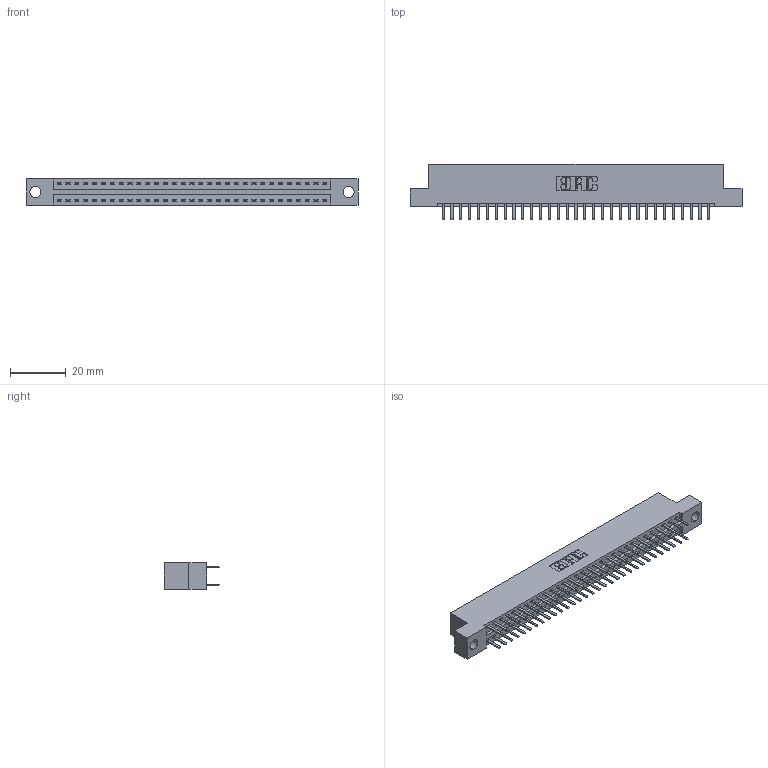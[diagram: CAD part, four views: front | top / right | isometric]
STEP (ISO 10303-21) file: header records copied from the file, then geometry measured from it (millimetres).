
FILE_DESCRIPTION (( 'STEP AP203' ), '1' );
FILE_NAME ('346-062-520-204.STEP', '2022-05-24T13:14:54', ( '' ), ( '' ), 'SwSTEP 2.0', 'SolidWorks 2020', '' );
FILE_SCHEMA (( 'CONFIG_CONTROL_DESIGN' ));
Length unit declared in the file: inch
Products named in the file (3): 345-292-001_345-293-120; 346-062-520-204; 346 Part_Flush Mounting Lugs - 0.156 Dia-TH
Assembly tree (63 placements, depth 2):
  346-062-520-204
    346 Part_Flush Mounting Lugs - 0.156 Dia-TH
    345-292-001_345-293-120  x62
Bounding box: 119 x 20.02 x 9.4 mm (x, y, z)
Volume: 11385.2 mm3; surface area: 15260.9 mm2
Topology: 63 solids, 63 shells, 3608 faces, 10471 edges, 6814 vertices
Faces by surface type: plane 2384, cylinder 1224
Entity records: 22245 total; most frequent: CARTESIAN_POINT 3698, ORIENTED_EDGE 3618, DIRECTION 3297, EDGE_CURVE 1809, VECTOR 1549, LINE 1549, VERTEX_POINT 1202, AXIS2_PLACEMENT_3D 874
